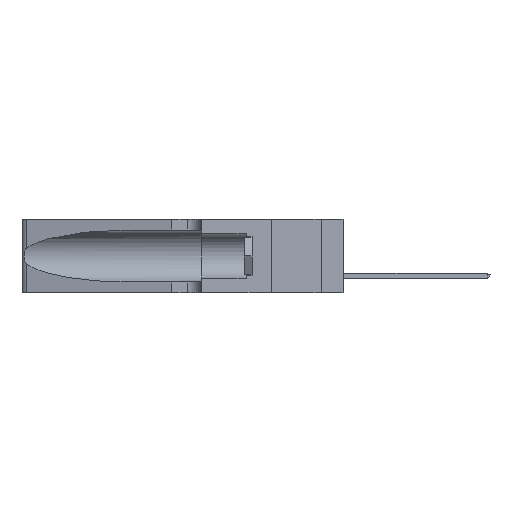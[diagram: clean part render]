
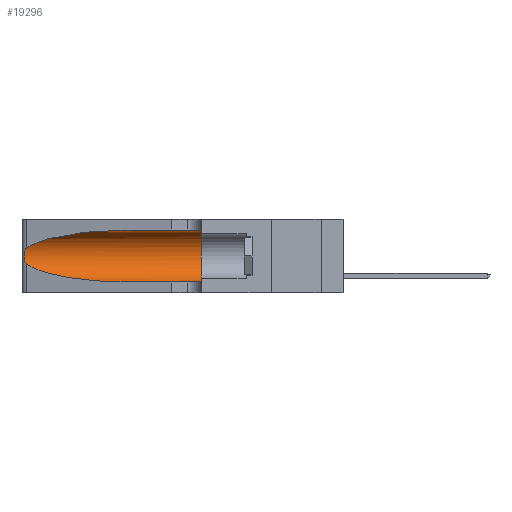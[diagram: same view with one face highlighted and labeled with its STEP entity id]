
A CAD part, left-side view. The second image highlights one B-rep face of the part: STEP entity #19296.
In plain terms, the highlighted cylindrical face has radius 3.308 mm (diameter 6.617 mm), a partial arc.
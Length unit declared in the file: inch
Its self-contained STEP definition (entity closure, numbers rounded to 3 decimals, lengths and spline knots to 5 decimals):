
#1577 = LINE ( 'NONE', #31437, #37965 ) ;
#1818 = DIRECTION ( 'NONE',  ( 0., 0., 1. ) ) ;
#2116 = DIRECTION ( 'NONE',  ( 0., -1., 0. ) ) ;
#2549 = VERTEX_POINT ( 'NONE', #27499 ) ;
#2800 = CARTESIAN_POINT ( 'NONE',  ( 0.26018, 1.23835, 0.19895 ) ) ;
#3259 = ORIENTED_EDGE ( 'NONE', *, *, #13717, .T. ) ;
#3267 = AXIS2_PLACEMENT_3D ( 'NONE', #30791, #11577, #1818 ) ;
#3398 = CARTESIAN_POINT ( 'NONE',  ( 0.1305, 0.35, 0.05475 ) ) ;
#3476 = ORIENTED_EDGE ( 'NONE', *, *, #9084, .T. ) ;
#3826 = CARTESIAN_POINT ( 'NONE',  ( 0.1305, 1.61858, 0.185 ) ) ;
#4879 = CARTESIAN_POINT ( 'NONE',  ( 0.25487, 1.22718, 0.22369 ) ) ;
#5034 = CARTESIAN_POINT ( 'NONE',  ( 0.2373, 1.15595, 0.28018 ) ) ;
#5656 = FACE_OUTER_BOUND ( 'NONE', #36876, .T. ) ;
#5947 = B_SPLINE_CURVE_WITH_KNOTS ( 'NONE', 3,
 ( #22341, #38719, #16019, #38854, #18789, #2800, #12528, #35597, #35471, #6104, #41573, #35038, #38298, #22045 ),
 .UNSPECIFIED., .F., .F.,
 ( 4, 2, 2, 2, 2, 2, 4 ),
 ( 0., 0.00027, 0.00053, 0.00107, 0.0016, 0.00187, 0.00214 ),
 .UNSPECIFIED. ) ;
#6104 = CARTESIAN_POINT ( 'NONE',  ( 0.25856, 1.23593, 0.16098 ) ) ;
#6214 = VECTOR ( 'NONE', #14659, 39.37008 ) ;
#6686 =( BOUNDED_CURVE ( )  B_SPLINE_CURVE ( 3, ( #30142, #33379, #5034, #4879 ),
 .UNSPECIFIED., .F., .F. ) 
 B_SPLINE_CURVE_WITH_KNOTS ( ( 4, 4 ),
 ( 1.5708, 2.84003 ),
 .UNSPECIFIED. ) 
 CURVE ( )  GEOMETRIC_REPRESENTATION_ITEM ( )  RATIONAL_B_SPLINE_CURVE ( ( 1., 0.87, 0.87, 1. ) ) 
 REPRESENTATION_ITEM ( '' )  );
#7356 = ORIENTED_EDGE ( 'NONE', *, *, #28439, .F. ) ;
#8018 = CARTESIAN_POINT ( 'NONE',  ( 0.25487, 1.22718, 0.22369 ) ) ;
#8263 = CARTESIAN_POINT ( 'NONE',  ( 0.25487, 1.22718, 0.14631 ) ) ;
#8978 = CARTESIAN_POINT ( 'NONE',  ( 0.1305, 0.35, 0.31525 ) ) ;
#9084 = EDGE_CURVE ( 'NONE', #37026, #2549, #5947, .T. ) ;
#9690 = VERTEX_POINT ( 'NONE', #3398 ) ;
#11379 = CARTESIAN_POINT ( 'NONE',  ( 0.1305, 1.61858, 0.05475 ) ) ;
#11395 = CARTESIAN_POINT ( 'NONE',  ( 0.1305, 0.72297, 0.05475 ) ) ;
#11521 = CARTESIAN_POINT ( 'NONE',  ( 0.1305, 0.72297, 0.31525 ) ) ;
#11577 = DIRECTION ( 'NONE',  ( 0., 1., 0. ) ) ;
#12364 = VERTEX_POINT ( 'NONE', #30626 ) ;
#12528 = CARTESIAN_POINT ( 'NONE',  ( 0.26075, 1.23896, 0.19203 ) ) ;
#12804 = ORIENTED_EDGE ( 'NONE', *, *, #33165, .T. ) ;
#13717 = EDGE_CURVE ( 'NONE', #2549, #12364, #22539, .T. ) ;
#14396 = LINE ( 'NONE', #11379, #6214 ) ;
#14659 = DIRECTION ( 'NONE',  ( 0., -1., 0. ) ) ;
#16019 = CARTESIAN_POINT ( 'NONE',  ( 0.25639, 1.23184, 0.21858 ) ) ;
#18789 = CARTESIAN_POINT ( 'NONE',  ( 0.25854, 1.2359, 0.20912 ) ) ;
#18887 = VERTEX_POINT ( 'NONE', #8978 ) ;
#19296 = ADVANCED_FACE ( 'NONE', ( #5656 ), #39887, .F. ) ;
#19727 = CIRCLE ( 'NONE', #3267, 0.13025 ) ;
#20082 = DIRECTION ( 'NONE',  ( 0., -1., 0. ) ) ;
#22045 = CARTESIAN_POINT ( 'NONE',  ( 0.25487, 1.22718, 0.14631 ) ) ;
#22341 = CARTESIAN_POINT ( 'NONE',  ( 0.25487, 1.22718, 0.22369 ) ) ;
#22539 =( BOUNDED_CURVE ( )  B_SPLINE_CURVE ( 3, ( #8263, #27749, #34439, #11395 ),
 .UNSPECIFIED., .F., .F. ) 
 B_SPLINE_CURVE_WITH_KNOTS ( ( 4, 4 ),
 ( 3.44316, 4.71239 ),
 .UNSPECIFIED. ) 
 CURVE ( )  GEOMETRIC_REPRESENTATION_ITEM ( )  RATIONAL_B_SPLINE_CURVE ( ( 1., 0.87, 0.87, 1. ) ) 
 REPRESENTATION_ITEM ( '' )  );
#24698 = VERTEX_POINT ( 'NONE', #11521 ) ;
#27499 = CARTESIAN_POINT ( 'NONE',  ( 0.25487, 1.22718, 0.14631 ) ) ;
#27749 = CARTESIAN_POINT ( 'NONE',  ( 0.2373, 1.15595, 0.08982 ) ) ;
#28439 = EDGE_CURVE ( 'NONE', #18887, #9690, #19727, .T. ) ;
#30097 = EDGE_CURVE ( 'NONE', #12364, #9690, #14396, .T. ) ;
#30142 = CARTESIAN_POINT ( 'NONE',  ( 0.1305, 0.72297, 0.31525 ) ) ;
#30196 = EDGE_CURVE ( 'NONE', #24698, #18887, #1577, .T. ) ;
#30626 = CARTESIAN_POINT ( 'NONE',  ( 0.1305, 0.72297, 0.05475 ) ) ;
#30791 = CARTESIAN_POINT ( 'NONE',  ( 0.1305, 0.35, 0.185 ) ) ;
#31437 = CARTESIAN_POINT ( 'NONE',  ( 0.1305, 1.61858, 0.31525 ) ) ;
#33165 = EDGE_CURVE ( 'NONE', #24698, #37026, #6686, .T. ) ;
#33379 = CARTESIAN_POINT ( 'NONE',  ( 0.18966, 0.96281, 0.31525 ) ) ;
#34439 = CARTESIAN_POINT ( 'NONE',  ( 0.18966, 0.96281, 0.05475 ) ) ;
#35038 = CARTESIAN_POINT ( 'NONE',  ( 0.25639, 1.23186, 0.15144 ) ) ;
#35471 = CARTESIAN_POINT ( 'NONE',  ( 0.26017, 1.23833, 0.17102 ) ) ;
#35597 = CARTESIAN_POINT ( 'NONE',  ( 0.26075, 1.23896, 0.178 ) ) ;
#36876 = EDGE_LOOP ( 'NONE', ( #12804, #3476, #3259, #40675, #7356, #38019 ) ) ;
#37026 = VERTEX_POINT ( 'NONE', #8018 ) ;
#37965 = VECTOR ( 'NONE', #2116, 39.37008 ) ;
#38019 = ORIENTED_EDGE ( 'NONE', *, *, #30196, .F. ) ;
#38298 = CARTESIAN_POINT ( 'NONE',  ( 0.25555, 1.22993, 0.14849 ) ) ;
#38719 = CARTESIAN_POINT ( 'NONE',  ( 0.25555, 1.22994, 0.2215 ) ) ;
#38854 = CARTESIAN_POINT ( 'NONE',  ( 0.25787, 1.23484, 0.2124 ) ) ;
#38946 = AXIS2_PLACEMENT_3D ( 'NONE', #3826, #20082, #40002 ) ;
#39887 = CYLINDRICAL_SURFACE ( 'NONE', #38946, 0.13025 ) ;
#40002 = DIRECTION ( 'NONE',  ( 0., 0., -1. ) ) ;
#40675 = ORIENTED_EDGE ( 'NONE', *, *, #30097, .T. ) ;
#41573 = CARTESIAN_POINT ( 'NONE',  ( 0.25789, 1.23486, 0.15765 ) ) ;
